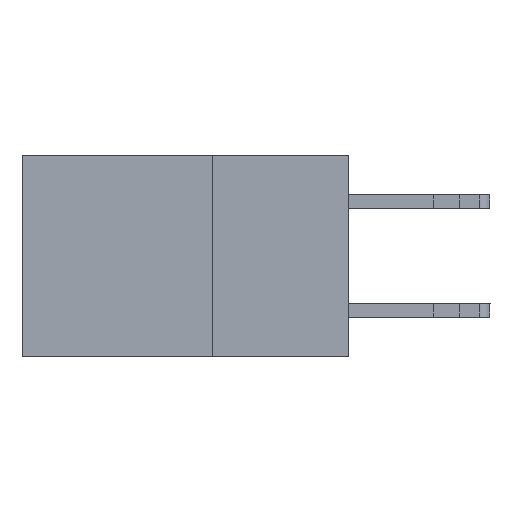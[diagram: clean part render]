
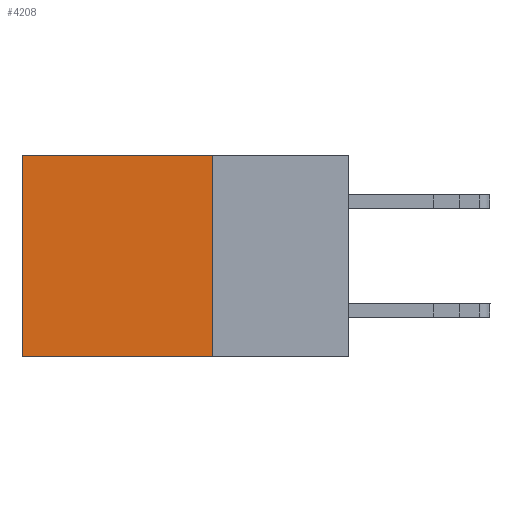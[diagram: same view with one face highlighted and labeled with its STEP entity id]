
A CAD part, left-side view. The second image highlights one B-rep face of the part: STEP entity #4208.
In plain terms, the highlighted planar face has unit normal (-1, 0, 0).
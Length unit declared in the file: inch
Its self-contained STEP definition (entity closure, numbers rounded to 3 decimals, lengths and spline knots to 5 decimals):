
#398 = VECTOR ( 'NONE', #11511, 39.37008 ) ;
#681 = LINE ( 'NONE', #4013, #11677 ) ;
#766 = AXIS2_PLACEMENT_3D ( 'NONE', #2857, #6697, #1908 ) ;
#1026 = LINE ( 'NONE', #2372, #11263 ) ;
#1145 = LINE ( 'NONE', #8559, #398 ) ;
#1260 = VECTOR ( 'NONE', #2558, 39.37008 ) ;
#1908 = DIRECTION ( 'NONE',  ( 0., 0., -1. ) ) ;
#2372 = CARTESIAN_POINT ( 'NONE',  ( 0.298, 0.25, -0.37 ) ) ;
#2516 = VERTEX_POINT ( 'NONE', #2831 ) ;
#2558 = DIRECTION ( 'NONE',  ( 0., 1., 0. ) ) ;
#2831 = CARTESIAN_POINT ( 'NONE',  ( 0.298, 0.6, -0.37 ) ) ;
#2857 = CARTESIAN_POINT ( 'NONE',  ( 0.298, 0.25, 0. ) ) ;
#3596 = DIRECTION ( 'NONE',  ( 0., 0., -1. ) ) ;
#3635 = LINE ( 'NONE', #8208, #1260 ) ;
#4013 = CARTESIAN_POINT ( 'NONE',  ( 0.298, 0.25, 0. ) ) ;
#4208 = ADVANCED_FACE ( 'NONE', ( #8084 ), #6654, .F. ) ;
#4592 = EDGE_CURVE ( 'NONE', #12347, #2516, #1026, .T. ) ;
#4602 = VERTEX_POINT ( 'NONE', #7118 ) ;
#6105 = ORIENTED_EDGE ( 'NONE', *, *, #7126, .T. ) ;
#6654 = PLANE ( 'NONE',  #766 ) ;
#6697 = DIRECTION ( 'NONE',  ( 1., 0., 0. ) ) ;
#7073 = ORIENTED_EDGE ( 'NONE', *, *, #10608, .T. ) ;
#7118 = CARTESIAN_POINT ( 'NONE',  ( 0.298, 0.6, 0. ) ) ;
#7126 = EDGE_CURVE ( 'NONE', #12132, #4602, #3635, .T. ) ;
#7337 = ORIENTED_EDGE ( 'NONE', *, *, #4592, .F. ) ;
#8002 = CARTESIAN_POINT ( 'NONE',  ( 0.298, 0.25, -0.37 ) ) ;
#8084 = FACE_OUTER_BOUND ( 'NONE', #11631, .T. ) ;
#8208 = CARTESIAN_POINT ( 'NONE',  ( 0.298, 0.25, 0. ) ) ;
#8413 = CARTESIAN_POINT ( 'NONE',  ( 0.298, 0.25, 0. ) ) ;
#8559 = CARTESIAN_POINT ( 'NONE',  ( 0.298, 0.6, 0. ) ) ;
#8994 = DIRECTION ( 'NONE',  ( 0., 1., 0. ) ) ;
#10403 = ORIENTED_EDGE ( 'NONE', *, *, #10803, .F. ) ;
#10608 = EDGE_CURVE ( 'NONE', #4602, #2516, #1145, .T. ) ;
#10803 = EDGE_CURVE ( 'NONE', #12132, #12347, #681, .T. ) ;
#11263 = VECTOR ( 'NONE', #8994, 39.37008 ) ;
#11511 = DIRECTION ( 'NONE',  ( 0., 0., -1. ) ) ;
#11631 = EDGE_LOOP ( 'NONE', ( #7073, #7337, #10403, #6105 ) ) ;
#11677 = VECTOR ( 'NONE', #3596, 39.37008 ) ;
#12132 = VERTEX_POINT ( 'NONE', #8413 ) ;
#12347 = VERTEX_POINT ( 'NONE', #8002 ) ;
